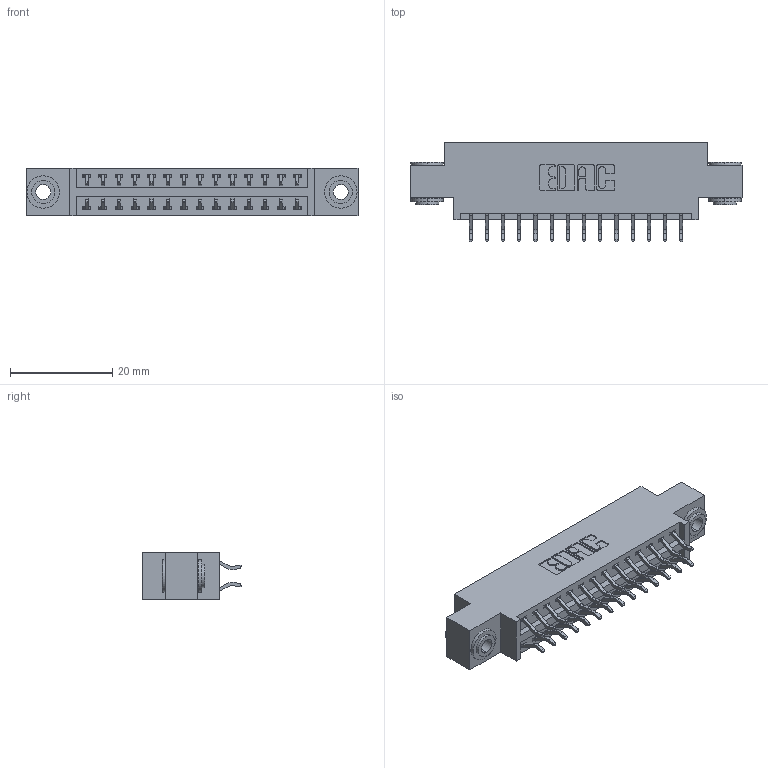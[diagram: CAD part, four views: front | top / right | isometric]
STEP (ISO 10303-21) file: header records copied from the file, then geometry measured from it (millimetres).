
FILE_DESCRIPTION (( 'STEP AP203' ), '1' );
FILE_NAME ('346-028-556-803.STEP', '2022-05-19T05:10:51', ( '' ), ( '' ), 'SwSTEP 2.0', 'SolidWorks 2020', '' );
FILE_SCHEMA (( 'CONFIG_CONTROL_DESIGN' ));
Length unit declared in the file: inch
Products named in the file (4): 346-028-556-803; 345-250-002_345-250-002-102; 346 Part_0.170 Offset - 0.156 Dia-TH; 345-292-001_556 Tail
Assembly tree (31 placements, depth 2):
  346-028-556-803
    346 Part_0.170 Offset - 0.156 Dia-TH
    345-292-001_556 Tail  x28
    345-250-002_345-250-002-102  x2
Bounding box: 65.02 x 19.57 x 9.4 mm (x, y, z)
Volume: 5968.8 mm3; surface area: 8166.7 mm2
Topology: 31 solids, 31 shells, 1802 faces, 5297 edges, 3490 vertices
Faces by surface type: plane 1196, cylinder 598, cone 8
Entity records: 14324 total; most frequent: CARTESIAN_POINT 2397, ORIENTED_EDGE 2310, DIRECTION 2181, EDGE_CURVE 1155, LINE 935, VECTOR 935, VERTEX_POINT 766, AXIS2_PLACEMENT_3D 623
